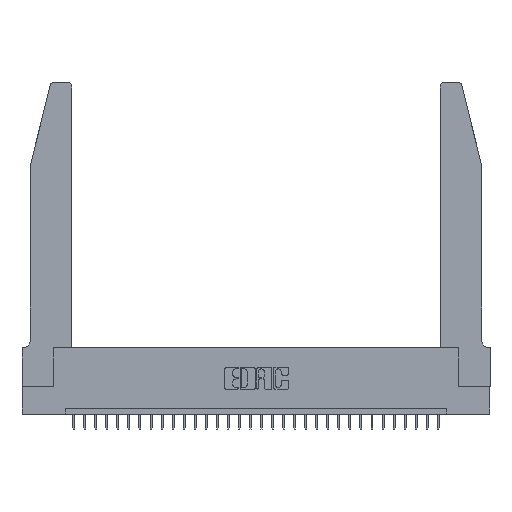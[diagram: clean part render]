
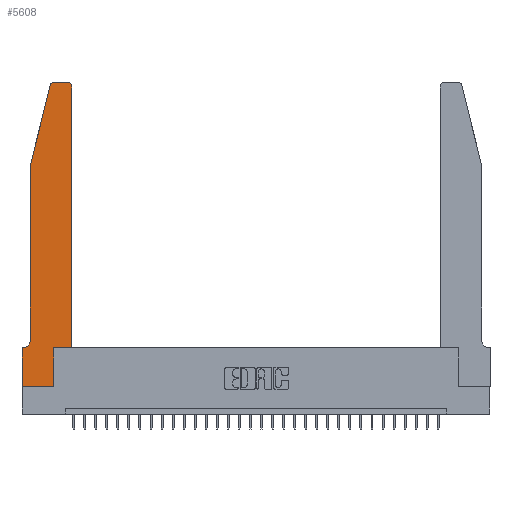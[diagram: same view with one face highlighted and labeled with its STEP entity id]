
A CAD part, top view. The second image highlights one B-rep face of the part: STEP entity #5608.
In plain terms, the highlighted planar face has unit normal (0, 0, 1).
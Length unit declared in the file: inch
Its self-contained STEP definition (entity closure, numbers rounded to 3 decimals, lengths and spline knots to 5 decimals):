
#101 = VECTOR ( 'NONE', #27219, 39.37008 ) ;
#107 = CARTESIAN_POINT ( 'NONE',  ( 0., 0., 0.37 ) ) ;
#1386 = AXIS2_PLACEMENT_3D ( 'NONE', #1804, #28412, #11528 ) ;
#1394 = ORIENTED_EDGE ( 'NONE', *, *, #16590, .T. ) ;
#1804 = CARTESIAN_POINT ( 'NONE',  ( 0.284, 2.72, 0.37 ) ) ;
#2370 = ORIENTED_EDGE ( 'NONE', *, *, #17423, .T. ) ;
#2723 = CARTESIAN_POINT ( 'NONE',  ( 0.0755, 0.42, 0.37 ) ) ;
#3253 = CARTESIAN_POINT ( 'NONE',  ( 0.284, 2.75, 0.37 ) ) ;
#3397 = VERTEX_POINT ( 'NONE', #21261 ) ;
#3415 = VERTEX_POINT ( 'NONE', #19661 ) ;
#4860 = LINE ( 'NONE', #14564, #15826 ) ;
#5083 = AXIS2_PLACEMENT_3D ( 'NONE', #8921, #18646, #16411 ) ;
#5378 = DIRECTION ( 'NONE',  ( 0., 0., -1. ) ) ;
#5489 = DIRECTION ( 'NONE',  ( 1., 0., 0. ) ) ;
#5513 = VECTOR ( 'NONE', #7132, 39.37008 ) ;
#5522 = VERTEX_POINT ( 'NONE', #3253 ) ;
#5608 = ADVANCED_FACE ( 'NONE', ( #22847 ), #5958, .T. ) ;
#5774 = CARTESIAN_POINT ( 'NONE',  ( 0.25487, 2.72718, 0.37 ) ) ;
#5779 = CARTESIAN_POINT ( 'NONE',  ( 0.2605, 2.75, 0.37 ) ) ;
#5958 = PLANE ( 'NONE',  #17929 ) ;
#6010 = VERTEX_POINT ( 'NONE', #27746 ) ;
#6054 = VECTOR ( 'NONE', #30143, 39.37008 ) ;
#7132 = DIRECTION ( 'NONE',  ( 1., 0., 0. ) ) ;
#7239 = LINE ( 'NONE', #31008, #19472 ) ;
#7781 = CARTESIAN_POINT ( 'NONE',  ( 0.0755, 2., 0.37 ) ) ;
#7924 = CARTESIAN_POINT ( 'NONE',  ( 0.2865, 0., 0.37 ) ) ;
#8052 = CIRCLE ( 'NONE', #20770, 0.07 ) ;
#8078 = DIRECTION ( 'NONE',  ( -1., 0., 0. ) ) ;
#8256 = ORIENTED_EDGE ( 'NONE', *, *, #19681, .T. ) ;
#8404 = EDGE_CURVE ( 'NONE', #14879, #12855, #14432, .T. ) ;
#8921 = CARTESIAN_POINT ( 'NONE',  ( 0.4205, 2.72, 0.37 ) ) ;
#9153 = LINE ( 'NONE', #28437, #28112 ) ;
#10560 = LINE ( 'NONE', #5779, #6054 ) ;
#10629 = CARTESIAN_POINT ( 'NONE',  ( 0.0055, 0.42, 0.37 ) ) ;
#11136 = CARTESIAN_POINT ( 'NONE',  ( 0.0055, 0.35, 0.37 ) ) ;
#11443 = DIRECTION ( 'NONE',  ( 0., -1., 0. ) ) ;
#11528 = DIRECTION ( 'NONE',  ( 1., 0., 0. ) ) ;
#11590 = EDGE_CURVE ( 'NONE', #12855, #3397, #20998, .T. ) ;
#12000 = CARTESIAN_POINT ( 'NONE',  ( 0., 0.35, 0.37 ) ) ;
#12026 = VERTEX_POINT ( 'NONE', #16934 ) ;
#12506 = VECTOR ( 'NONE', #11443, 39.37008 ) ;
#12855 = VERTEX_POINT ( 'NONE', #12000 ) ;
#12996 = VERTEX_POINT ( 'NONE', #5774 ) ;
#13948 = VERTEX_POINT ( 'NONE', #7924 ) ;
#14432 = LINE ( 'NONE', #21914, #28201 ) ;
#14564 = CARTESIAN_POINT ( 'NONE',  ( 0.4505, 0.35, 0.37 ) ) ;
#14879 = VERTEX_POINT ( 'NONE', #11136 ) ;
#15128 = CIRCLE ( 'NONE', #1386, 0.03 ) ;
#15298 = ORIENTED_EDGE ( 'NONE', *, *, #29165, .T. ) ;
#15340 = VERTEX_POINT ( 'NONE', #18748 ) ;
#15515 = DIRECTION ( 'NONE',  ( 1., 0., 0. ) ) ;
#15826 = VECTOR ( 'NONE', #15515, 39.37008 ) ;
#16020 = DIRECTION ( 'NONE',  ( 0., 1., 0. ) ) ;
#16068 = LINE ( 'NONE', #30085, #17544 ) ;
#16411 = DIRECTION ( 'NONE',  ( 1., 0., 0. ) ) ;
#16590 = EDGE_CURVE ( 'NONE', #5522, #12996, #15128, .T. ) ;
#16934 = CARTESIAN_POINT ( 'NONE',  ( 0.2865, 0.35, 0.37 ) ) ;
#16958 = DIRECTION ( 'NONE',  ( 0., 1., 0. ) ) ;
#17423 = EDGE_CURVE ( 'NONE', #3397, #13948, #29426, .T. ) ;
#17544 = VECTOR ( 'NONE', #28007, 39.37008 ) ;
#17929 = AXIS2_PLACEMENT_3D ( 'NONE', #20146, #29853, #5489 ) ;
#18144 = ORIENTED_EDGE ( 'NONE', *, *, #24217, .T. ) ;
#18393 = CIRCLE ( 'NONE', #5083, 0.03 ) ;
#18646 = DIRECTION ( 'NONE',  ( 0., 0., 1. ) ) ;
#18748 = CARTESIAN_POINT ( 'NONE',  ( 0.4205, 2.75, 0.37 ) ) ;
#18831 = EDGE_CURVE ( 'NONE', #29379, #14879, #8052, .T. ) ;
#19472 = VECTOR ( 'NONE', #16958, 39.37008 ) ;
#19661 = CARTESIAN_POINT ( 'NONE',  ( 0.4505, 2.72, 0.37 ) ) ;
#19681 = EDGE_CURVE ( 'NONE', #15340, #5522, #10560, .T. ) ;
#20146 = CARTESIAN_POINT ( 'NONE',  ( 0., 0.35, 0.37 ) ) ;
#20705 = EDGE_LOOP ( 'NONE', ( #8256, #1394, #21716, #26951, #31350, #23908, #22175, #2370, #26253, #15298, #18144, #30627 ) ) ;
#20770 = AXIS2_PLACEMENT_3D ( 'NONE', #10629, #5378, #8078 ) ;
#20998 = LINE ( 'NONE', #28331, #12506 ) ;
#21261 = CARTESIAN_POINT ( 'NONE',  ( 0., 0., 0.37 ) ) ;
#21716 = ORIENTED_EDGE ( 'NONE', *, *, #23928, .T. ) ;
#21914 = CARTESIAN_POINT ( 'NONE',  ( 0.0755, 0.35, 0.37 ) ) ;
#22175 = ORIENTED_EDGE ( 'NONE', *, *, #11590, .T. ) ;
#22847 = FACE_OUTER_BOUND ( 'NONE', #20705, .T. ) ;
#23908 = ORIENTED_EDGE ( 'NONE', *, *, #8404, .T. ) ;
#23928 = EDGE_CURVE ( 'NONE', #12996, #25266, #29600, .T. ) ;
#24217 = EDGE_CURVE ( 'NONE', #6010, #3415, #7239, .T. ) ;
#25266 = VERTEX_POINT ( 'NONE', #26935 ) ;
#25789 = EDGE_CURVE ( 'NONE', #13948, #12026, #9153, .T. ) ;
#26253 = ORIENTED_EDGE ( 'NONE', *, *, #25789, .T. ) ;
#26935 = CARTESIAN_POINT ( 'NONE',  ( 0.0755, 2., 0.37 ) ) ;
#26951 = ORIENTED_EDGE ( 'NONE', *, *, #27972, .T. ) ;
#27219 = DIRECTION ( 'NONE',  ( -0.239, -0.971, 0. ) ) ;
#27746 = CARTESIAN_POINT ( 'NONE',  ( 0.4505, 0.35, 0.37 ) ) ;
#27972 = EDGE_CURVE ( 'NONE', #25266, #29379, #16068, .T. ) ;
#28007 = DIRECTION ( 'NONE',  ( 0., -1., 0. ) ) ;
#28112 = VECTOR ( 'NONE', #16020, 39.37008 ) ;
#28201 = VECTOR ( 'NONE', #28922, 39.37008 ) ;
#28331 = CARTESIAN_POINT ( 'NONE',  ( 0., 0., 0.37 ) ) ;
#28412 = DIRECTION ( 'NONE',  ( 0., 0., 1. ) ) ;
#28437 = CARTESIAN_POINT ( 'NONE',  ( 0.2865, 0.35, 0.37 ) ) ;
#28922 = DIRECTION ( 'NONE',  ( -1., 0., 0. ) ) ;
#29165 = EDGE_CURVE ( 'NONE', #12026, #6010, #4860, .T. ) ;
#29379 = VERTEX_POINT ( 'NONE', #2723 ) ;
#29426 = LINE ( 'NONE', #107, #5513 ) ;
#29600 = LINE ( 'NONE', #7781, #101 ) ;
#29698 = EDGE_CURVE ( 'NONE', #3415, #15340, #18393, .T. ) ;
#29853 = DIRECTION ( 'NONE',  ( 0., 0., 1. ) ) ;
#30085 = CARTESIAN_POINT ( 'NONE',  ( 0.0755, 2., 0.37 ) ) ;
#30143 = DIRECTION ( 'NONE',  ( -1., 0., 0. ) ) ;
#30627 = ORIENTED_EDGE ( 'NONE', *, *, #29698, .T. ) ;
#31008 = CARTESIAN_POINT ( 'NONE',  ( 0.4505, 0.35, 0.37 ) ) ;
#31350 = ORIENTED_EDGE ( 'NONE', *, *, #18831, .T. ) ;
